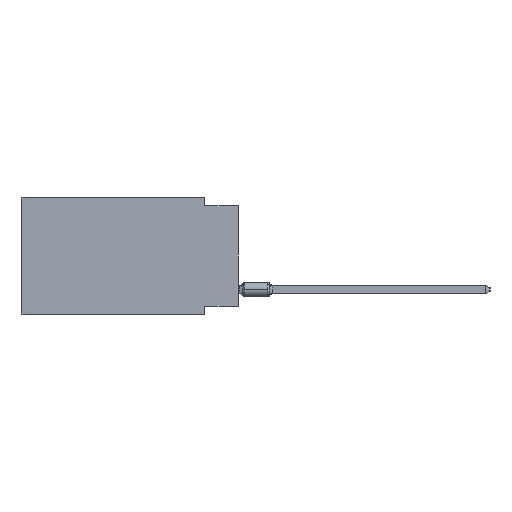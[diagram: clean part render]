
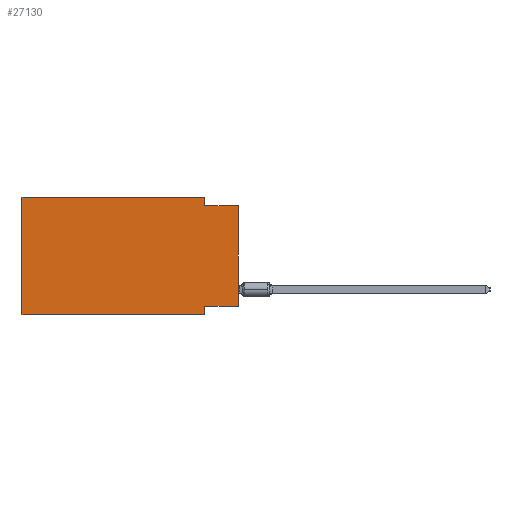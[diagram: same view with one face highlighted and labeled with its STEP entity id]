
A CAD part, left-side view. The second image highlights one B-rep face of the part: STEP entity #27130.
In plain terms, the highlighted planar face has unit normal (-1, 0, 0).
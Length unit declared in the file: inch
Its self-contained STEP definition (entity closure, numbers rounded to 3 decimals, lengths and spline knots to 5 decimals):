
#560 = EDGE_CURVE ( 'NONE', #33031, #19827, #8483, .T. ) ;
#771 = CARTESIAN_POINT ( 'NONE',  ( 0., 0.1, 0. ) ) ;
#1216 = ORIENTED_EDGE ( 'NONE', *, *, #18030, .F. ) ;
#1543 = CARTESIAN_POINT ( 'NONE',  ( 0., 0., -0.025 ) ) ;
#2020 = CARTESIAN_POINT ( 'NONE',  ( 0., 0.1, -0.35 ) ) ;
#2148 = LINE ( 'NONE', #25576, #18554 ) ;
#2839 = ORIENTED_EDGE ( 'NONE', *, *, #27373, .F. ) ;
#3223 = CARTESIAN_POINT ( 'NONE',  ( 0., 0.645, 0. ) ) ;
#3710 = VECTOR ( 'NONE', #33197, 39.37008 ) ;
#3757 = VECTOR ( 'NONE', #18929, 39.37008 ) ;
#3830 = LINE ( 'NONE', #771, #33284 ) ;
#3910 = CARTESIAN_POINT ( 'NONE',  ( 0., 0., -0.025 ) ) ;
#5081 = VECTOR ( 'NONE', #8437, 39.37008 ) ;
#6007 = EDGE_CURVE ( 'NONE', #32749, #15868, #17006, .T. ) ;
#6629 = DIRECTION ( 'NONE',  ( 0., -1., 0. ) ) ;
#7392 = CARTESIAN_POINT ( 'NONE',  ( 0., 0.645, 0. ) ) ;
#7718 = LINE ( 'NONE', #33537, #3710 ) ;
#8437 = DIRECTION ( 'NONE',  ( 0., 0., 1. ) ) ;
#8483 = LINE ( 'NONE', #3223, #20150 ) ;
#10700 = ORIENTED_EDGE ( 'NONE', *, *, #560, .F. ) ;
#11074 = EDGE_LOOP ( 'NONE', ( #31488, #24121, #11981, #10700, #2839, #25777, #1216, #12045 ) ) ;
#11981 = ORIENTED_EDGE ( 'NONE', *, *, #16726, .F. ) ;
#11982 = DIRECTION ( 'NONE',  ( 1., 0., 0. ) ) ;
#12045 = ORIENTED_EDGE ( 'NONE', *, *, #19875, .F. ) ;
#12318 = FACE_OUTER_BOUND ( 'NONE', #11074, .T. ) ;
#12375 = LINE ( 'NONE', #2020, #27930 ) ;
#12578 = VERTEX_POINT ( 'NONE', #17841 ) ;
#13204 = LINE ( 'NONE', #23576, #5081 ) ;
#13644 = VERTEX_POINT ( 'NONE', #29092 ) ;
#13648 = LINE ( 'NONE', #16539, #3757 ) ;
#14674 = EDGE_CURVE ( 'NONE', #20314, #12578, #7718, .T. ) ;
#15868 = VERTEX_POINT ( 'NONE', #3910 ) ;
#16464 = DIRECTION ( 'NONE',  ( 0., -1., 0. ) ) ;
#16539 = CARTESIAN_POINT ( 'NONE',  ( 0., 0.645, 0. ) ) ;
#16726 = EDGE_CURVE ( 'NONE', #19827, #32749, #3830, .T. ) ;
#17006 = LINE ( 'NONE', #1543, #31683 ) ;
#17760 = DIRECTION ( 'NONE',  ( 0., 0., -1. ) ) ;
#17841 = CARTESIAN_POINT ( 'NONE',  ( 0., 0.1, -0.35 ) ) ;
#18030 = EDGE_CURVE ( 'NONE', #13644, #12578, #12375, .T. ) ;
#18554 = VECTOR ( 'NONE', #33397, 39.37008 ) ;
#18929 = DIRECTION ( 'NONE',  ( 0., 0., 1. ) ) ;
#18953 = DIRECTION ( 'NONE',  ( 0., 0., -1. ) ) ;
#19827 = VERTEX_POINT ( 'NONE', #32725 ) ;
#19875 = EDGE_CURVE ( 'NONE', #30731, #13644, #2148, .T. ) ;
#20150 = VECTOR ( 'NONE', #16464, 39.37008 ) ;
#20314 = VERTEX_POINT ( 'NONE', #33013 ) ;
#22186 = EDGE_CURVE ( 'NONE', #30731, #15868, #13204, .T. ) ;
#23102 = DIRECTION ( 'NONE',  ( 0., 0., -1. ) ) ;
#23576 = CARTESIAN_POINT ( 'NONE',  ( 0., 0., 0. ) ) ;
#23784 = AXIS2_PLACEMENT_3D ( 'NONE', #7392, #11982, #17760 ) ;
#24121 = ORIENTED_EDGE ( 'NONE', *, *, #6007, .F. ) ;
#25576 = CARTESIAN_POINT ( 'NONE',  ( 0., 0., -0.325 ) ) ;
#25777 = ORIENTED_EDGE ( 'NONE', *, *, #14674, .T. ) ;
#27130 = ADVANCED_FACE ( 'NONE', ( #12318 ), #30668, .F. ) ;
#27373 = EDGE_CURVE ( 'NONE', #20314, #33031, #13648, .T. ) ;
#27930 = VECTOR ( 'NONE', #23102, 39.37008 ) ;
#28932 = CARTESIAN_POINT ( 'NONE',  ( 0., 0., -0.325 ) ) ;
#29092 = CARTESIAN_POINT ( 'NONE',  ( 0., 0.1, -0.325 ) ) ;
#30668 = PLANE ( 'NONE',  #23784 ) ;
#30731 = VERTEX_POINT ( 'NONE', #28932 ) ;
#31293 = CARTESIAN_POINT ( 'NONE',  ( 0., 0.645, 0. ) ) ;
#31488 = ORIENTED_EDGE ( 'NONE', *, *, #22186, .T. ) ;
#31668 = CARTESIAN_POINT ( 'NONE',  ( 0., 0.1, -0.025 ) ) ;
#31683 = VECTOR ( 'NONE', #6629, 39.37008 ) ;
#32725 = CARTESIAN_POINT ( 'NONE',  ( 0., 0.1, 0. ) ) ;
#32749 = VERTEX_POINT ( 'NONE', #31668 ) ;
#33013 = CARTESIAN_POINT ( 'NONE',  ( 0., 0.645, -0.35 ) ) ;
#33031 = VERTEX_POINT ( 'NONE', #31293 ) ;
#33197 = DIRECTION ( 'NONE',  ( 0., -1., 0. ) ) ;
#33284 = VECTOR ( 'NONE', #18953, 39.37008 ) ;
#33397 = DIRECTION ( 'NONE',  ( 0., 1., 0. ) ) ;
#33537 = CARTESIAN_POINT ( 'NONE',  ( 0., 0.645, -0.35 ) ) ;
